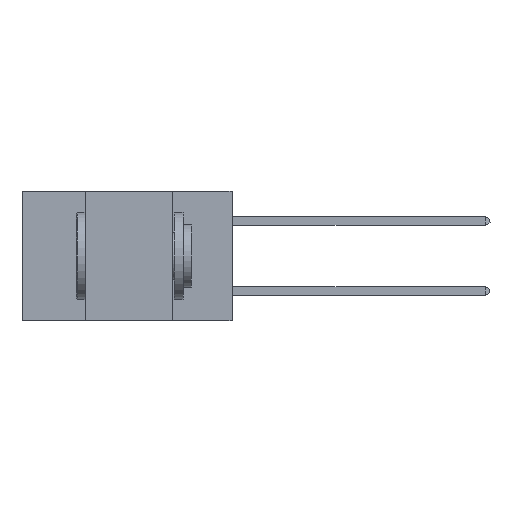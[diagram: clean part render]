
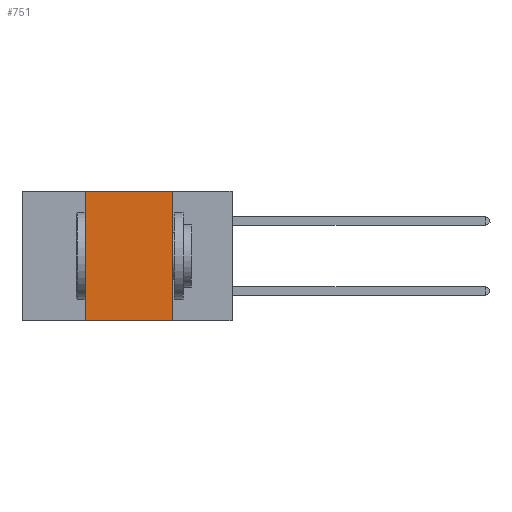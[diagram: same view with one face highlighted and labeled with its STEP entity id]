
A CAD part, left-side view. The second image highlights one B-rep face of the part: STEP entity #751.
In plain terms, the highlighted planar face has unit normal (-1, 0, 0).
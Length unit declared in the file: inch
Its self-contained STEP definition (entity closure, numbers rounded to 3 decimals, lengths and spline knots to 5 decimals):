
#88 = EDGE_CURVE ( 'NONE', #1748, #18370, #7386, .T. ) ;
#422 = CARTESIAN_POINT ( 'NONE',  ( 0., 0.42, -0.37 ) ) ;
#751 = ADVANCED_FACE ( 'NONE', ( #9359 ), #1101, .F. ) ;
#1101 = PLANE ( 'NONE',  #9050 ) ;
#1165 = EDGE_CURVE ( 'NONE', #12660, #1748, #19832, .T. ) ;
#1420 = CARTESIAN_POINT ( 'NONE',  ( 0., 0.6, 0. ) ) ;
#1748 = VERTEX_POINT ( 'NONE', #11046 ) ;
#1796 = EDGE_CURVE ( 'NONE', #18370, #13132, #6099, .T. ) ;
#2764 = CARTESIAN_POINT ( 'NONE',  ( 0., 0.42, 0. ) ) ;
#4557 = DIRECTION ( 'NONE',  ( 0., -1., 0. ) ) ;
#5011 = EDGE_LOOP ( 'NONE', ( #16145, #14589, #12632, #17892 ) ) ;
#5577 = VECTOR ( 'NONE', #10325, 39.37008 ) ;
#5719 = DIRECTION ( 'NONE',  ( 0., 0., -1. ) ) ;
#6099 = LINE ( 'NONE', #14592, #5577 ) ;
#7386 = LINE ( 'NONE', #1420, #18122 ) ;
#9050 = AXIS2_PLACEMENT_3D ( 'NONE', #10728, #13943, #5719 ) ;
#9359 = FACE_OUTER_BOUND ( 'NONE', #5011, .T. ) ;
#10325 = DIRECTION ( 'NONE',  ( 0., 0., -1. ) ) ;
#10581 = VECTOR ( 'NONE', #20364, 39.37008 ) ;
#10728 = CARTESIAN_POINT ( 'NONE',  ( 0., 0.6, 0. ) ) ;
#11046 = CARTESIAN_POINT ( 'NONE',  ( 0., 0.42, 0. ) ) ;
#11301 = CARTESIAN_POINT ( 'NONE',  ( 0., 0.17, 0. ) ) ;
#12397 = EDGE_CURVE ( 'NONE', #12660, #13132, #18085, .T. ) ;
#12632 = ORIENTED_EDGE ( 'NONE', *, *, #1165, .F. ) ;
#12660 = VERTEX_POINT ( 'NONE', #422 ) ;
#13132 = VERTEX_POINT ( 'NONE', #18890 ) ;
#13835 = VECTOR ( 'NONE', #14650, 39.37008 ) ;
#13943 = DIRECTION ( 'NONE',  ( 1., 0., 0. ) ) ;
#14589 = ORIENTED_EDGE ( 'NONE', *, *, #88, .F. ) ;
#14592 = CARTESIAN_POINT ( 'NONE',  ( 0., 0.17, 0. ) ) ;
#14650 = DIRECTION ( 'NONE',  ( 0., -1., 0. ) ) ;
#16145 = ORIENTED_EDGE ( 'NONE', *, *, #1796, .F. ) ;
#16367 = CARTESIAN_POINT ( 'NONE',  ( 0., 0.6, -0.37 ) ) ;
#17892 = ORIENTED_EDGE ( 'NONE', *, *, #12397, .T. ) ;
#18085 = LINE ( 'NONE', #16367, #13835 ) ;
#18122 = VECTOR ( 'NONE', #4557, 39.37008 ) ;
#18370 = VERTEX_POINT ( 'NONE', #11301 ) ;
#18890 = CARTESIAN_POINT ( 'NONE',  ( 0., 0.17, -0.37 ) ) ;
#19832 = LINE ( 'NONE', #2764, #10581 ) ;
#20364 = DIRECTION ( 'NONE',  ( 0., 0., 1. ) ) ;
